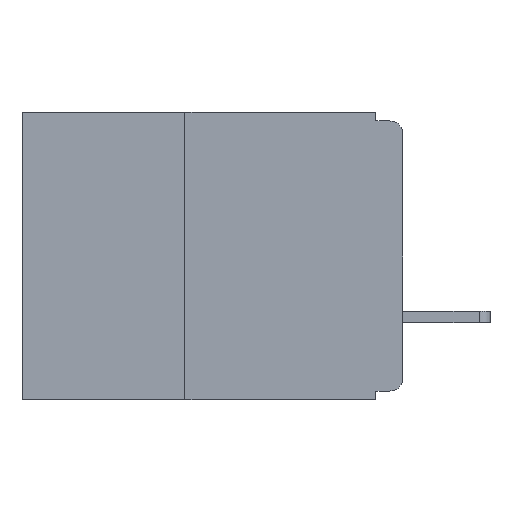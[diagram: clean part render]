
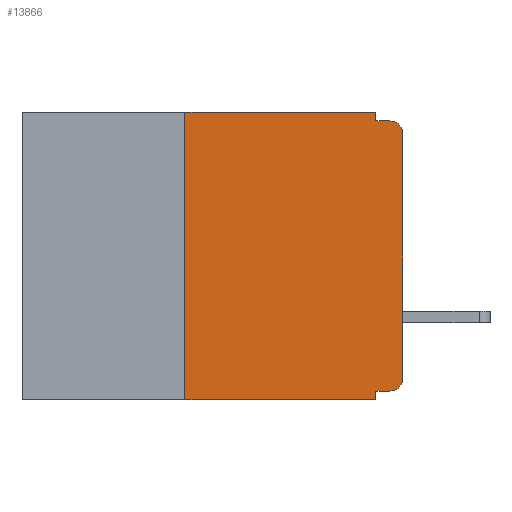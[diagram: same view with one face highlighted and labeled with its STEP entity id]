
A CAD part, left-side view. The second image highlights one B-rep face of the part: STEP entity #13866.
In plain terms, the highlighted planar face has unit normal (-1, 0, 0).
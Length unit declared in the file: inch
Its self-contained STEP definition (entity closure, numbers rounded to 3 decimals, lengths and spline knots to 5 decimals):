
#149 = EDGE_CURVE ( 'NONE', #739, #22040, #3441, .T. ) ;
#196 = VERTEX_POINT ( 'NONE', #24127 ) ;
#321 = VECTOR ( 'NONE', #17473, 39.37008 ) ;
#739 = VERTEX_POINT ( 'NONE', #23926 ) ;
#802 = LINE ( 'NONE', #17155, #25656 ) ;
#1216 = ORIENTED_EDGE ( 'NONE', *, *, #28115, .F. ) ;
#2425 = CIRCLE ( 'NONE', #11707, 0.015 ) ;
#2580 = CARTESIAN_POINT ( 'NONE',  ( 0., 0.437, 0. ) ) ;
#2632 = CARTESIAN_POINT ( 'NONE',  ( 0., 0.031, -0.33 ) ) ;
#3249 = VERTEX_POINT ( 'NONE', #6590 ) ;
#3441 = LINE ( 'NONE', #30693, #15530 ) ;
#3755 = AXIS2_PLACEMENT_3D ( 'NONE', #24998, #10749, #27359 ) ;
#4416 = DIRECTION ( 'NONE',  ( 0., 1., 0. ) ) ;
#4667 = DIRECTION ( 'NONE',  ( 0., -1., 0. ) ) ;
#5108 = VERTEX_POINT ( 'NONE', #2632 ) ;
#5342 = VERTEX_POINT ( 'NONE', #21183 ) ;
#6029 = EDGE_CURVE ( 'NONE', #13094, #5108, #802, .T. ) ;
#6317 = CIRCLE ( 'NONE', #21834, 0.015 ) ;
#6401 = ORIENTED_EDGE ( 'NONE', *, *, #29129, .F. ) ;
#6590 = CARTESIAN_POINT ( 'NONE',  ( 0., 0.031, -0.32 ) ) ;
#6684 = LINE ( 'NONE', #9766, #25013 ) ;
#6762 = DIRECTION ( 'NONE',  ( 0., 0., -1. ) ) ;
#7436 = VECTOR ( 'NONE', #4416, 39.37008 ) ;
#7890 = VECTOR ( 'NONE', #4667, 39.37008 ) ;
#7929 = VERTEX_POINT ( 'NONE', #17458 ) ;
#8236 = ORIENTED_EDGE ( 'NONE', *, *, #16340, .F. ) ;
#8794 = CARTESIAN_POINT ( 'NONE',  ( 0., 0.015, -0.025 ) ) ;
#9201 = DIRECTION ( 'NONE',  ( 0., 0., -1. ) ) ;
#9766 = CARTESIAN_POINT ( 'NONE',  ( 0., 0.031, -0.33 ) ) ;
#10749 = DIRECTION ( 'NONE',  ( 1., 0., 0. ) ) ;
#11210 = DIRECTION ( 'NONE',  ( 0., 0., -1. ) ) ;
#11707 = AXIS2_PLACEMENT_3D ( 'NONE', #28373, #23464, #9201 ) ;
#11893 = VECTOR ( 'NONE', #19422, 39.37008 ) ;
#12198 = DIRECTION ( 'NONE',  ( 0., 0., -1. ) ) ;
#12719 = DIRECTION ( 'NONE',  ( 0., 0., 1. ) ) ;
#12727 = CARTESIAN_POINT ( 'NONE',  ( 0., 0.25, -0.33 ) ) ;
#12841 = EDGE_CURVE ( 'NONE', #14394, #5342, #26698, .T. ) ;
#13094 = VERTEX_POINT ( 'NONE', #14974 ) ;
#13866 = ADVANCED_FACE ( 'NONE', ( #22943 ), #22599, .F. ) ;
#14394 = VERTEX_POINT ( 'NONE', #22354 ) ;
#14775 = ORIENTED_EDGE ( 'NONE', *, *, #30787, .T. ) ;
#14974 = CARTESIAN_POINT ( 'NONE',  ( 0., 0.25, -0.33 ) ) ;
#15255 = CARTESIAN_POINT ( 'NONE',  ( 0., 0., -0.025 ) ) ;
#15530 = VECTOR ( 'NONE', #12719, 39.37008 ) ;
#15583 = VECTOR ( 'NONE', #6762, 39.37008 ) ;
#16340 = EDGE_CURVE ( 'NONE', #3249, #5108, #6684, .T. ) ;
#16789 = DIRECTION ( 'NONE',  ( 0., -1., 0. ) ) ;
#17155 = CARTESIAN_POINT ( 'NONE',  ( 0., 0.437, -0.33 ) ) ;
#17458 = CARTESIAN_POINT ( 'NONE',  ( 0., 0.25, 0. ) ) ;
#17473 = DIRECTION ( 'NONE',  ( 0., 0., 1. ) ) ;
#18492 = EDGE_CURVE ( 'NONE', #7929, #14394, #25289, .T. ) ;
#19422 = DIRECTION ( 'NONE',  ( 0., -1., 0. ) ) ;
#20152 = LINE ( 'NONE', #28222, #7436 ) ;
#20943 = ORIENTED_EDGE ( 'NONE', *, *, #18492, .F. ) ;
#21101 = CARTESIAN_POINT ( 'NONE',  ( 0., 0.031, 0. ) ) ;
#21183 = CARTESIAN_POINT ( 'NONE',  ( 0., 0.031, -0.01 ) ) ;
#21247 = ORIENTED_EDGE ( 'NONE', *, *, #29104, .T. ) ;
#21834 = AXIS2_PLACEMENT_3D ( 'NONE', #8794, #25442, #11210 ) ;
#22040 = VERTEX_POINT ( 'NONE', #15255 ) ;
#22354 = CARTESIAN_POINT ( 'NONE',  ( 0., 0.031, 0. ) ) ;
#22462 = VERTEX_POINT ( 'NONE', #26326 ) ;
#22599 = PLANE ( 'NONE',  #3755 ) ;
#22647 = ORIENTED_EDGE ( 'NONE', *, *, #12841, .F. ) ;
#22943 = FACE_OUTER_BOUND ( 'NONE', #24193, .T. ) ;
#23464 = DIRECTION ( 'NONE',  ( -1., 0., 0. ) ) ;
#23926 = CARTESIAN_POINT ( 'NONE',  ( 0., 0., -0.305 ) ) ;
#24127 = CARTESIAN_POINT ( 'NONE',  ( 0., 0.015, -0.01 ) ) ;
#24193 = EDGE_LOOP ( 'NONE', ( #27705, #14775, #1216, #22647, #20943, #30960, #25476, #8236, #6401, #21247 ) ) ;
#24802 = EDGE_CURVE ( 'NONE', #13094, #7929, #25958, .T. ) ;
#24998 = CARTESIAN_POINT ( 'NONE',  ( 0., 0.437, 0. ) ) ;
#25013 = VECTOR ( 'NONE', #12198, 39.37008 ) ;
#25289 = LINE ( 'NONE', #2580, #11893 ) ;
#25442 = DIRECTION ( 'NONE',  ( -1., 0., 0. ) ) ;
#25476 = ORIENTED_EDGE ( 'NONE', *, *, #6029, .T. ) ;
#25656 = VECTOR ( 'NONE', #16789, 39.37008 ) ;
#25958 = LINE ( 'NONE', #12727, #321 ) ;
#26326 = CARTESIAN_POINT ( 'NONE',  ( 0., 0.015, -0.32 ) ) ;
#26698 = LINE ( 'NONE', #21101, #15583 ) ;
#26903 = LINE ( 'NONE', #30796, #7890 ) ;
#27359 = DIRECTION ( 'NONE',  ( 0., 0., -1. ) ) ;
#27705 = ORIENTED_EDGE ( 'NONE', *, *, #149, .T. ) ;
#28115 = EDGE_CURVE ( 'NONE', #5342, #196, #26903, .T. ) ;
#28222 = CARTESIAN_POINT ( 'NONE',  ( 0., 0., -0.32 ) ) ;
#28373 = CARTESIAN_POINT ( 'NONE',  ( 0., 0.015, -0.305 ) ) ;
#29104 = EDGE_CURVE ( 'NONE', #22462, #739, #2425, .T. ) ;
#29129 = EDGE_CURVE ( 'NONE', #22462, #3249, #20152, .T. ) ;
#30693 = CARTESIAN_POINT ( 'NONE',  ( 0., 0., 0. ) ) ;
#30787 = EDGE_CURVE ( 'NONE', #22040, #196, #6317, .T. ) ;
#30796 = CARTESIAN_POINT ( 'NONE',  ( 0., 0., -0.01 ) ) ;
#30960 = ORIENTED_EDGE ( 'NONE', *, *, #24802, .F. ) ;
